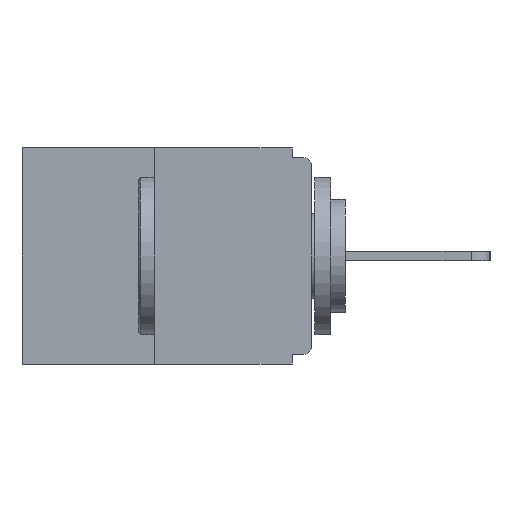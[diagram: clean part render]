
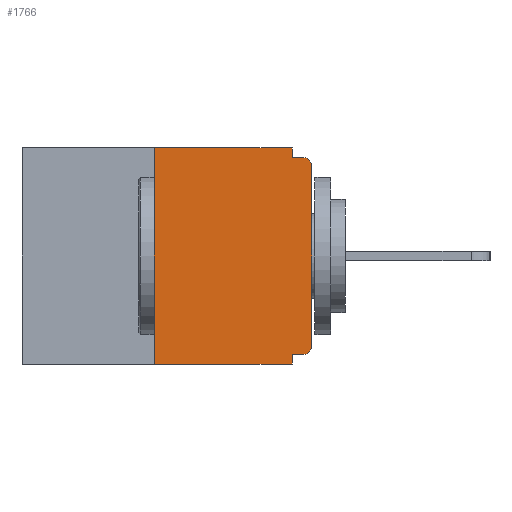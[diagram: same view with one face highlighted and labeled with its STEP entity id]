
A CAD part, left-side view. The second image highlights one B-rep face of the part: STEP entity #1766.
In plain terms, the highlighted planar face has unit normal (-1, 0, 0).
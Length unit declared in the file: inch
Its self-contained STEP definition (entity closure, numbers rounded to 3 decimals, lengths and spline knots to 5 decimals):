
#65 = CARTESIAN_POINT ( 'NONE',  ( 0., 0., -0.313 ) ) ;
#123 = DIRECTION ( 'NONE',  ( -1., 0., 0. ) ) ;
#363 = LINE ( 'NONE', #7852, #9727 ) ;
#584 = LINE ( 'NONE', #9194, #7373 ) ;
#933 = LINE ( 'NONE', #8119, #4136 ) ;
#1015 = EDGE_CURVE ( 'NONE', #12241, #9725, #8370, .T. ) ;
#1543 = ORIENTED_EDGE ( 'NONE', *, *, #9505, .T. ) ;
#1766 = ADVANCED_FACE ( 'NONE', ( #4842 ), #9484, .F. ) ;
#1853 = EDGE_CURVE ( 'NONE', #6530, #9725, #6171, .T. ) ;
#2023 = ORIENTED_EDGE ( 'NONE', *, *, #10591, .F. ) ;
#2189 = VERTEX_POINT ( 'NONE', #3054 ) ;
#2229 = DIRECTION ( 'NONE',  ( 0., 0., -1. ) ) ;
#2255 = CARTESIAN_POINT ( 'NONE',  ( 0., 0.031, -0.343 ) ) ;
#2878 = VECTOR ( 'NONE', #11477, 39.37008 ) ;
#3025 = VECTOR ( 'NONE', #8569, 39.37008 ) ;
#3054 = CARTESIAN_POINT ( 'NONE',  ( 0., 0.031, -0.015 ) ) ;
#3080 = ORIENTED_EDGE ( 'NONE', *, *, #14458, .T. ) ;
#3550 = DIRECTION ( 'NONE',  ( 0., 0., -1. ) ) ;
#3648 = ORIENTED_EDGE ( 'NONE', *, *, #8783, .F. ) ;
#3722 = AXIS2_PLACEMENT_3D ( 'NONE', #7763, #123, #8876 ) ;
#3909 = ORIENTED_EDGE ( 'NONE', *, *, #9814, .T. ) ;
#4136 = VECTOR ( 'NONE', #9227, 39.37008 ) ;
#4197 = CARTESIAN_POINT ( 'NONE',  ( 0., 0.031, 0. ) ) ;
#4842 = FACE_OUTER_BOUND ( 'NONE', #5796, .T. ) ;
#4881 = ORIENTED_EDGE ( 'NONE', *, *, #1853, .T. ) ;
#5161 = CIRCLE ( 'NONE', #11809, 0.015 ) ;
#5198 = DIRECTION ( 'NONE',  ( 0., 0., -1. ) ) ;
#5230 = DIRECTION ( 'NONE',  ( -1., 0., 0. ) ) ;
#5253 = CARTESIAN_POINT ( 'NONE',  ( 0., 0.015, -0.313 ) ) ;
#5317 = VECTOR ( 'NONE', #2229, 39.37008 ) ;
#5411 = VERTEX_POINT ( 'NONE', #13336 ) ;
#5756 = VERTEX_POINT ( 'NONE', #4197 ) ;
#5796 = EDGE_LOOP ( 'NONE', ( #11116, #10003, #4881, #11647, #13257, #3909, #1543, #3080, #2023, #3648 ) ) ;
#6094 = CARTESIAN_POINT ( 'NONE',  ( 0., 0.46, 0. ) ) ;
#6111 = CARTESIAN_POINT ( 'NONE',  ( 0., 0.031, -0.343 ) ) ;
#6171 = LINE ( 'NONE', #12319, #2878 ) ;
#6530 = VERTEX_POINT ( 'NONE', #7463 ) ;
#7279 = VERTEX_POINT ( 'NONE', #13565 ) ;
#7324 = DIRECTION ( 'NONE',  ( 0., -1., 0. ) ) ;
#7373 = VECTOR ( 'NONE', #9181, 39.37008 ) ;
#7382 = VERTEX_POINT ( 'NONE', #11997 ) ;
#7450 = VERTEX_POINT ( 'NONE', #10723 ) ;
#7463 = CARTESIAN_POINT ( 'NONE',  ( 0., 0.25, -0.343 ) ) ;
#7763 = CARTESIAN_POINT ( 'NONE',  ( 0., 0.015, -0.03 ) ) ;
#7852 = CARTESIAN_POINT ( 'NONE',  ( 0., 0., 0. ) ) ;
#7867 = DIRECTION ( 'NONE',  ( 0., 0., 1. ) ) ;
#8084 = VERTEX_POINT ( 'NONE', #65 ) ;
#8119 = CARTESIAN_POINT ( 'NONE',  ( 0., 0.46, 0. ) ) ;
#8235 = CIRCLE ( 'NONE', #3722, 0.015 ) ;
#8370 = LINE ( 'NONE', #2255, #5317 ) ;
#8569 = DIRECTION ( 'NONE',  ( 0., 0., 1. ) ) ;
#8655 = CARTESIAN_POINT ( 'NONE',  ( 0., 0.25, 0. ) ) ;
#8783 = EDGE_CURVE ( 'NONE', #5756, #2189, #14245, .T. ) ;
#8876 = DIRECTION ( 'NONE',  ( 0., 0., -1. ) ) ;
#9181 = DIRECTION ( 'NONE',  ( 0., 1., 0. ) ) ;
#9194 = CARTESIAN_POINT ( 'NONE',  ( 0., 0., -0.328 ) ) ;
#9227 = DIRECTION ( 'NONE',  ( 0., -1., 0. ) ) ;
#9256 = EDGE_CURVE ( 'NONE', #5411, #12241, #584, .T. ) ;
#9339 = EDGE_CURVE ( 'NONE', #6530, #7382, #14232, .T. ) ;
#9484 = PLANE ( 'NONE',  #13244 ) ;
#9505 = EDGE_CURVE ( 'NONE', #8084, #7279, #363, .T. ) ;
#9725 = VERTEX_POINT ( 'NONE', #6111 ) ;
#9727 = VECTOR ( 'NONE', #7867, 39.37008 ) ;
#9814 = EDGE_CURVE ( 'NONE', #5411, #8084, #5161, .T. ) ;
#10003 = ORIENTED_EDGE ( 'NONE', *, *, #9339, .F. ) ;
#10331 = VECTOR ( 'NONE', #7324, 39.37008 ) ;
#10591 = EDGE_CURVE ( 'NONE', #2189, #7450, #13000, .T. ) ;
#10723 = CARTESIAN_POINT ( 'NONE',  ( 0., 0.015, -0.015 ) ) ;
#11116 = ORIENTED_EDGE ( 'NONE', *, *, #12695, .F. ) ;
#11289 = DIRECTION ( 'NONE',  ( 0., 0., -1. ) ) ;
#11333 = CARTESIAN_POINT ( 'NONE',  ( 0., 0.031, 0. ) ) ;
#11477 = DIRECTION ( 'NONE',  ( 0., -1., 0. ) ) ;
#11604 = VECTOR ( 'NONE', #11289, 39.37008 ) ;
#11647 = ORIENTED_EDGE ( 'NONE', *, *, #1015, .F. ) ;
#11809 = AXIS2_PLACEMENT_3D ( 'NONE', #5253, #5230, #5198 ) ;
#11997 = CARTESIAN_POINT ( 'NONE',  ( 0., 0.25, 0. ) ) ;
#12241 = VERTEX_POINT ( 'NONE', #13578 ) ;
#12319 = CARTESIAN_POINT ( 'NONE',  ( 0., 0.46, -0.343 ) ) ;
#12695 = EDGE_CURVE ( 'NONE', #7382, #5756, #933, .T. ) ;
#13000 = LINE ( 'NONE', #13486, #10331 ) ;
#13244 = AXIS2_PLACEMENT_3D ( 'NONE', #6094, #13901, #3550 ) ;
#13257 = ORIENTED_EDGE ( 'NONE', *, *, #9256, .F. ) ;
#13336 = CARTESIAN_POINT ( 'NONE',  ( 0., 0.015, -0.328 ) ) ;
#13486 = CARTESIAN_POINT ( 'NONE',  ( 0., 0., -0.015 ) ) ;
#13565 = CARTESIAN_POINT ( 'NONE',  ( 0., 0., -0.03 ) ) ;
#13578 = CARTESIAN_POINT ( 'NONE',  ( 0., 0.031, -0.328 ) ) ;
#13901 = DIRECTION ( 'NONE',  ( 1., 0., 0. ) ) ;
#14232 = LINE ( 'NONE', #8655, #3025 ) ;
#14245 = LINE ( 'NONE', #11333, #11604 ) ;
#14458 = EDGE_CURVE ( 'NONE', #7279, #7450, #8235, .T. ) ;
